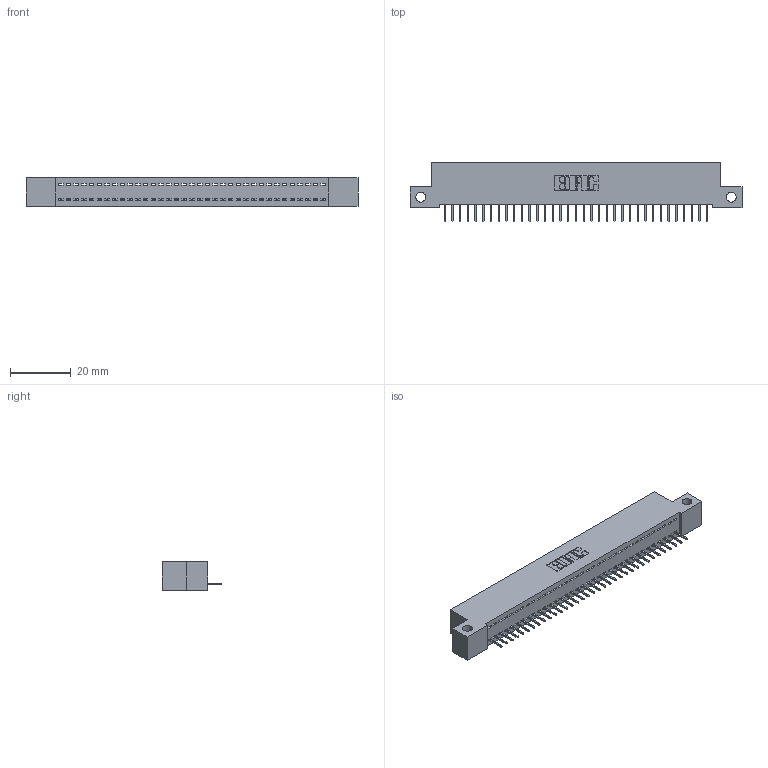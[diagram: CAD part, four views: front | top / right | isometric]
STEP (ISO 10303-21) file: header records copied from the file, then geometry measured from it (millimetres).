
FILE_DESCRIPTION (( 'STEP AP203' ), '1' );
FILE_NAME ('342-035-524-112.STEP', '2018-08-11T19:25:58', ( '' ), ( '' ), 'SwSTEP 2.0', 'SolidWorks 2016', '' );
FILE_SCHEMA (( 'CONFIG_CONTROL_DESIGN' ));
Length unit declared in the file: inch
Products named in the file (3): 342-035-524-112; 342 Part_Side Mount; 345-292-001_345-293-124
Assembly tree (36 placements, depth 2):
  342-035-524-112
    342 Part_Side Mount
    345-292-001_345-293-124  x35
Bounding box: 109.22 x 19.69 x 9.4 mm (x, y, z)
Volume: 9338.4 mm3; surface area: 12989.8 mm2
Topology: 36 solids, 36 shells, 2280 faces, 6599 edges, 4258 vertices
Faces by surface type: plane 1746, cylinder 534
Entity records: 22247 total; most frequent: CARTESIAN_POINT 3843, ORIENTED_EDGE 3814, DIRECTION 3257, EDGE_CURVE 1907, VECTOR 1783, LINE 1783, VERTEX_POINT 1266, AXIS2_PLACEMENT_3D 737
